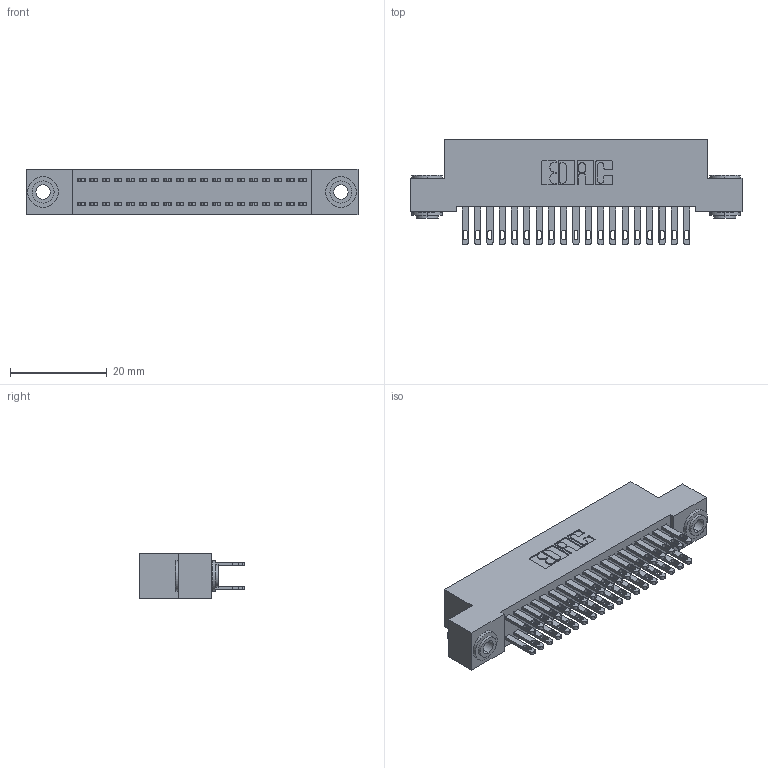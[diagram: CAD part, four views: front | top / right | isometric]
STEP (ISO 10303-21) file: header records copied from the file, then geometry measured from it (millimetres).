
FILE_DESCRIPTION (( 'STEP AP203' ), '1' );
FILE_NAME ('342-038-500-203.STEP', '2018-08-11T21:41:17', ( '' ), ( '' ), 'SwSTEP 2.0', 'SolidWorks 2016', '' );
FILE_SCHEMA (( 'CONFIG_CONTROL_DESIGN' ));
Length unit declared in the file: inch
Products named in the file (4): 342 Part_.156 TH; 345-292-001_345-293-100; 342-250-002_345-250-002-102; 342-038-500-203
Assembly tree (41 placements, depth 2):
  342-038-500-203
    342 Part_.156 TH
    345-292-001_345-293-100  x38
    342-250-002_345-250-002-102  x2
Bounding box: 68.58 x 21.85 x 9.4 mm (x, y, z)
Volume: 6192 mm3; surface area: 10090.2 mm2
Topology: 41 solids, 41 shells, 1972 faces, 5961 edges, 3970 vertices
Faces by surface type: plane 1216, cylinder 748, cone 8
Entity records: 15646 total; most frequent: CARTESIAN_POINT 2593, ORIENTED_EDGE 2522, DIRECTION 2291, EDGE_CURVE 1261, LINE 1105, VECTOR 1105, VERTEX_POINT 838, AXIS2_PLACEMENT_3D 593
